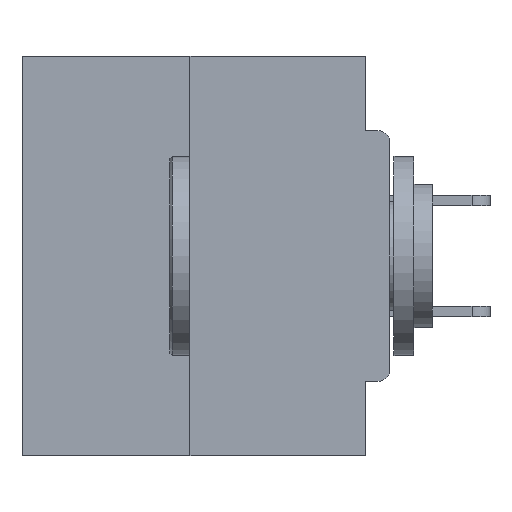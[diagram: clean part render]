
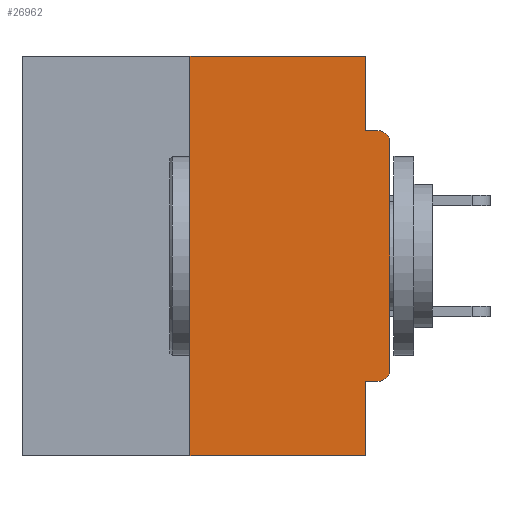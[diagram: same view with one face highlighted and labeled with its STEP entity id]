
A CAD part, left-side view. The second image highlights one B-rep face of the part: STEP entity #26962.
In plain terms, the highlighted planar face has unit normal (-1, 0, 0).
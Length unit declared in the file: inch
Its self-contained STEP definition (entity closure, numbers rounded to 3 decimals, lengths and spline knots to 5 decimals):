
#744 = CARTESIAN_POINT ( 'NONE',  ( 0., 0.015, -0.3915 ) ) ;
#938 = ORIENTED_EDGE ( 'NONE', *, *, #33008, .F. ) ;
#1106 = ORIENTED_EDGE ( 'NONE', *, *, #6286, .F. ) ;
#2349 = CARTESIAN_POINT ( 'NONE',  ( 0., 0.015, -0.1085 ) ) ;
#3485 = DIRECTION ( 'NONE',  ( 0., -1., 0. ) ) ;
#3593 = DIRECTION ( 'NONE',  ( -1., 0., 0. ) ) ;
#4173 = CARTESIAN_POINT ( 'NONE',  ( 0., 0.031, -0.4065 ) ) ;
#4204 = DIRECTION ( 'NONE',  ( 0., 0., -1. ) ) ;
#4301 = VERTEX_POINT ( 'NONE', #24439 ) ;
#4401 = CARTESIAN_POINT ( 'NONE',  ( 0., 0.031, 0. ) ) ;
#5286 = ORIENTED_EDGE ( 'NONE', *, *, #22949, .T. ) ;
#5526 = ORIENTED_EDGE ( 'NONE', *, *, #35356, .F. ) ;
#6286 = EDGE_CURVE ( 'NONE', #19363, #21241, #27368, .T. ) ;
#6551 = LINE ( 'NONE', #12653, #29271 ) ;
#7754 = CARTESIAN_POINT ( 'NONE',  ( 0., 0.25, 0. ) ) ;
#8024 = LINE ( 'NONE', #26296, #25782 ) ;
#9141 = AXIS2_PLACEMENT_3D ( 'NONE', #12631, #35761, #4204 ) ;
#10036 = CARTESIAN_POINT ( 'NONE',  ( 0., 0.25, 0. ) ) ;
#10635 = AXIS2_PLACEMENT_3D ( 'NONE', #2349, #22171, #25007 ) ;
#12085 = EDGE_CURVE ( 'NONE', #20504, #16417, #23328, .T. ) ;
#12254 = CARTESIAN_POINT ( 'NONE',  ( 0., 0., -0.0935 ) ) ;
#12631 = CARTESIAN_POINT ( 'NONE',  ( 0., 0.46, 0. ) ) ;
#12653 = CARTESIAN_POINT ( 'NONE',  ( 0., 0.031, -0.5 ) ) ;
#12757 = VECTOR ( 'NONE', #14046, 39.37008 ) ;
#14046 = DIRECTION ( 'NONE',  ( 0., -1., 0. ) ) ;
#15195 = ORIENTED_EDGE ( 'NONE', *, *, #34963, .F. ) ;
#15883 = VERTEX_POINT ( 'NONE', #19660 ) ;
#16417 = VERTEX_POINT ( 'NONE', #32195 ) ;
#16485 = EDGE_CURVE ( 'NONE', #4301, #20504, #8024, .T. ) ;
#16894 = ORIENTED_EDGE ( 'NONE', *, *, #16485, .T. ) ;
#17012 = CARTESIAN_POINT ( 'NONE',  ( 0., 0.031, 0. ) ) ;
#17675 = EDGE_CURVE ( 'NONE', #25273, #16417, #19912, .T. ) ;
#17717 = VECTOR ( 'NONE', #32445, 39.37008 ) ;
#18916 = VECTOR ( 'NONE', #26882, 39.37008 ) ;
#19004 = LINE ( 'NONE', #17012, #25258 ) ;
#19071 = CARTESIAN_POINT ( 'NONE',  ( 0., 0.031, -0.5 ) ) ;
#19363 = VERTEX_POINT ( 'NONE', #19523 ) ;
#19523 = CARTESIAN_POINT ( 'NONE',  ( 0., 0.015, -0.4065 ) ) ;
#19660 = CARTESIAN_POINT ( 'NONE',  ( 0., 0.25, -0.5 ) ) ;
#19912 = LINE ( 'NONE', #12254, #17717 ) ;
#19979 = VECTOR ( 'NONE', #36208, 39.37008 ) ;
#20504 = VERTEX_POINT ( 'NONE', #23045 ) ;
#20739 = FACE_OUTER_BOUND ( 'NONE', #22517, .T. ) ;
#21241 = VERTEX_POINT ( 'NONE', #4173 ) ;
#21765 = VERTEX_POINT ( 'NONE', #4401 ) ;
#21768 = LINE ( 'NONE', #7754, #19979 ) ;
#22171 = DIRECTION ( 'NONE',  ( -1., 0., 0. ) ) ;
#22517 = EDGE_LOOP ( 'NONE', ( #24846, #15195, #29259, #5526, #1106, #5286, #16894, #29987, #23064, #938 ) ) ;
#22583 = VERTEX_POINT ( 'NONE', #19071 ) ;
#22718 = LINE ( 'NONE', #26171, #29807 ) ;
#22949 = EDGE_CURVE ( 'NONE', #19363, #4301, #25883, .T. ) ;
#23045 = CARTESIAN_POINT ( 'NONE',  ( 0., 0., -0.1085 ) ) ;
#23064 = ORIENTED_EDGE ( 'NONE', *, *, #17675, .F. ) ;
#23328 = CIRCLE ( 'NONE', #10635, 0.015 ) ;
#23449 = LINE ( 'NONE', #28170, #12757 ) ;
#24439 = CARTESIAN_POINT ( 'NONE',  ( 0., 0., -0.3915 ) ) ;
#24846 = ORIENTED_EDGE ( 'NONE', *, *, #31358, .F. ) ;
#24969 = DIRECTION ( 'NONE',  ( 0., 0., -1. ) ) ;
#25007 = DIRECTION ( 'NONE',  ( 0., 0., -1. ) ) ;
#25258 = VECTOR ( 'NONE', #24969, 39.37008 ) ;
#25273 = VERTEX_POINT ( 'NONE', #26698 ) ;
#25782 = VECTOR ( 'NONE', #29792, 39.37008 ) ;
#25883 = CIRCLE ( 'NONE', #29782, 0.015 ) ;
#26171 = CARTESIAN_POINT ( 'NONE',  ( 0., 0.46, 0. ) ) ;
#26296 = CARTESIAN_POINT ( 'NONE',  ( 0., 0., 0. ) ) ;
#26442 = DIRECTION ( 'NONE',  ( 0., 0., -1. ) ) ;
#26698 = CARTESIAN_POINT ( 'NONE',  ( 0., 0.031, -0.0935 ) ) ;
#26882 = DIRECTION ( 'NONE',  ( 0., 1., 0. ) ) ;
#26962 = ADVANCED_FACE ( 'NONE', ( #20739 ), #30038, .F. ) ;
#27368 = LINE ( 'NONE', #35711, #18916 ) ;
#28170 = CARTESIAN_POINT ( 'NONE',  ( 0., 0.46, -0.5 ) ) ;
#29259 = ORIENTED_EDGE ( 'NONE', *, *, #33954, .T. ) ;
#29271 = VECTOR ( 'NONE', #26442, 39.37008 ) ;
#29275 = DIRECTION ( 'NONE',  ( 0., 0., -1. ) ) ;
#29782 = AXIS2_PLACEMENT_3D ( 'NONE', #744, #3593, #29275 ) ;
#29792 = DIRECTION ( 'NONE',  ( 0., 0., 1. ) ) ;
#29807 = VECTOR ( 'NONE', #3485, 39.37008 ) ;
#29987 = ORIENTED_EDGE ( 'NONE', *, *, #12085, .T. ) ;
#30038 = PLANE ( 'NONE',  #9141 ) ;
#31358 = EDGE_CURVE ( 'NONE', #36041, #21765, #22718, .T. ) ;
#32195 = CARTESIAN_POINT ( 'NONE',  ( 0., 0.015, -0.0935 ) ) ;
#32445 = DIRECTION ( 'NONE',  ( 0., -1., 0. ) ) ;
#33008 = EDGE_CURVE ( 'NONE', #21765, #25273, #19004, .T. ) ;
#33954 = EDGE_CURVE ( 'NONE', #15883, #22583, #23449, .T. ) ;
#34963 = EDGE_CURVE ( 'NONE', #15883, #36041, #21768, .T. ) ;
#35356 = EDGE_CURVE ( 'NONE', #21241, #22583, #6551, .T. ) ;
#35711 = CARTESIAN_POINT ( 'NONE',  ( 0., 0., -0.4065 ) ) ;
#35761 = DIRECTION ( 'NONE',  ( 1., 0., 0. ) ) ;
#36041 = VERTEX_POINT ( 'NONE', #10036 ) ;
#36208 = DIRECTION ( 'NONE',  ( 0., 0., 1. ) ) ;
